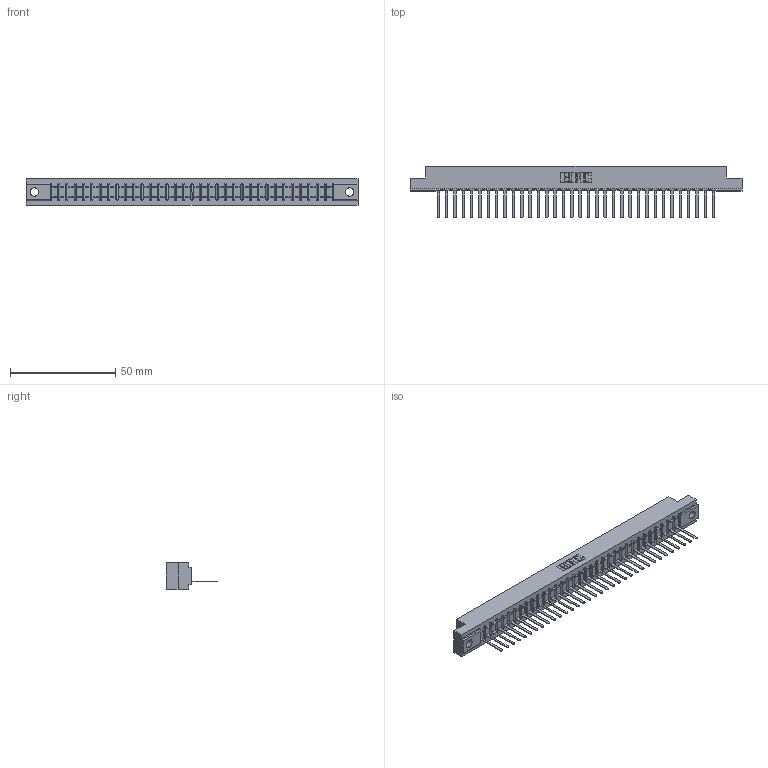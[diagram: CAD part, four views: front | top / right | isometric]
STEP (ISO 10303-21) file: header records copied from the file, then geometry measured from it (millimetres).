
FILE_DESCRIPTION (( 'STEP AP203' ), '1' );
FILE_NAME ('307-034-441-104.STEP', '2020-09-28T21:25:44', ( '' ), ( '' ), 'SwSTEP 2.0', 'SolidWorks 2020', '' );
FILE_SCHEMA (( 'CONFIG_CONTROL_DESIGN' ));
Length unit declared in the file: inch
Products named in the file (3): 307-290-002_541; 307 Part_.156 Dia Mounting Holes; 307-034-441-104
Assembly tree (35 placements, depth 2):
  307-034-441-104
    307 Part_.156 Dia Mounting Holes
    307-290-002_541  x34
Bounding box: 157.73 x 24.59 x 12.7 mm (x, y, z)
Volume: 16809.9 mm3; surface area: 21414.2 mm2
Topology: 35 solids, 35 shells, 2683 faces, 8247 edges, 5402 vertices
Faces by surface type: plane 1614, cylinder 999, sphere 70
Entity records: 31270 total; most frequent: CARTESIAN_POINT 5278, ORIENTED_EDGE 5266, DIRECTION 5123, EDGE_CURVE 2633, VECTOR 2021, LINE 2021, VERTEX_POINT 1706, AXIS2_PLACEMENT_3D 1551
